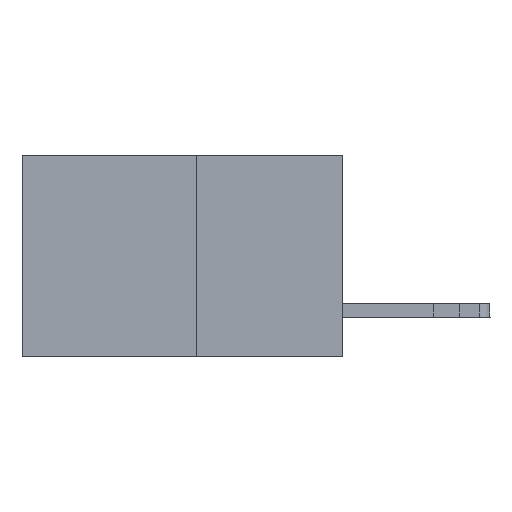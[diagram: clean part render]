
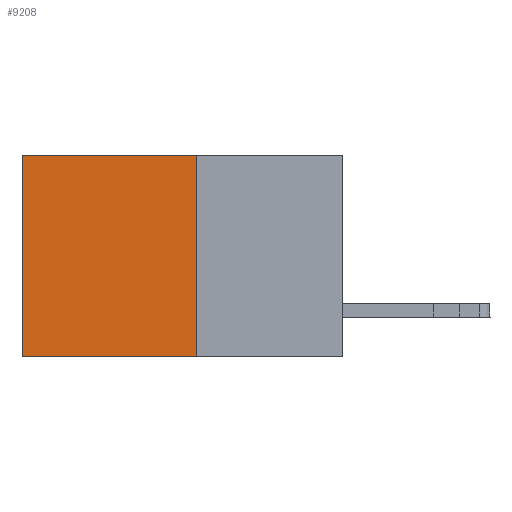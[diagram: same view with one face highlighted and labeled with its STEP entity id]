
A CAD part, left-side view. The second image highlights one B-rep face of the part: STEP entity #9208.
In plain terms, the highlighted planar face has unit normal (-1, 0, 0).
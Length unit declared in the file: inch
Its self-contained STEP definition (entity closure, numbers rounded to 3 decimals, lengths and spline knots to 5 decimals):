
#609 = VERTEX_POINT ( 'NONE', #3076 ) ;
#2181 = CARTESIAN_POINT ( 'NONE',  ( 0.277, 0.27, -0.37 ) ) ;
#3076 = CARTESIAN_POINT ( 'NONE',  ( 0.277, 0.59, 0. ) ) ;
#3656 = LINE ( 'NONE', #2181, #8646 ) ;
#4742 = EDGE_CURVE ( 'NONE', #609, #24808, #18990, .T. ) ;
#4834 = VECTOR ( 'NONE', #27083, 39.37008 ) ;
#4889 = CARTESIAN_POINT ( 'NONE',  ( 0.277, 0.27, -0.37 ) ) ;
#5163 = CARTESIAN_POINT ( 'NONE',  ( 0.277, 0.27, -0.37 ) ) ;
#5278 = VERTEX_POINT ( 'NONE', #5163 ) ;
#5493 = CARTESIAN_POINT ( 'NONE',  ( 0.277, 0.27, 0. ) ) ;
#5925 = ORIENTED_EDGE ( 'NONE', *, *, #21394, .F. ) ;
#7027 = DIRECTION ( 'NONE',  ( 0., 0., -1. ) ) ;
#7408 = CARTESIAN_POINT ( 'NONE',  ( 0.277, 0.59, -0.37 ) ) ;
#8122 = AXIS2_PLACEMENT_3D ( 'NONE', #4889, #19868, #7027 ) ;
#8646 = VECTOR ( 'NONE', #12830, 39.37008 ) ;
#9208 = ADVANCED_FACE ( 'NONE', ( #23493 ), #15577, .F. ) ;
#9570 = CARTESIAN_POINT ( 'NONE',  ( 0.277, 0.27, 0. ) ) ;
#10059 = CARTESIAN_POINT ( 'NONE',  ( 0.277, 0.27, -0.37 ) ) ;
#11189 = LINE ( 'NONE', #10059, #4834 ) ;
#12830 = DIRECTION ( 'NONE',  ( 0., 1., 0. ) ) ;
#13363 = LINE ( 'NONE', #5493, #18428 ) ;
#13367 = EDGE_CURVE ( 'NONE', #5278, #24808, #3656, .T. ) ;
#15577 = PLANE ( 'NONE',  #8122 ) ;
#16421 = EDGE_LOOP ( 'NONE', ( #23532, #22009, #5925, #22046 ) ) ;
#18428 = VECTOR ( 'NONE', #26819, 39.37008 ) ;
#18990 = LINE ( 'NONE', #25886, #25272 ) ;
#19868 = DIRECTION ( 'NONE',  ( 1., 0., 0. ) ) ;
#21394 = EDGE_CURVE ( 'NONE', #21914, #5278, #11189, .T. ) ;
#21914 = VERTEX_POINT ( 'NONE', #9570 ) ;
#22009 = ORIENTED_EDGE ( 'NONE', *, *, #13367, .F. ) ;
#22046 = ORIENTED_EDGE ( 'NONE', *, *, #24205, .T. ) ;
#23493 = FACE_OUTER_BOUND ( 'NONE', #16421, .T. ) ;
#23532 = ORIENTED_EDGE ( 'NONE', *, *, #4742, .T. ) ;
#24205 = EDGE_CURVE ( 'NONE', #21914, #609, #13363, .T. ) ;
#24808 = VERTEX_POINT ( 'NONE', #7408 ) ;
#25272 = VECTOR ( 'NONE', #25728, 39.37008 ) ;
#25728 = DIRECTION ( 'NONE',  ( 0., 0., -1. ) ) ;
#25886 = CARTESIAN_POINT ( 'NONE',  ( 0.277, 0.59, -0.37 ) ) ;
#26819 = DIRECTION ( 'NONE',  ( 0., 1., 0. ) ) ;
#27083 = DIRECTION ( 'NONE',  ( 0., 0., -1. ) ) ;
